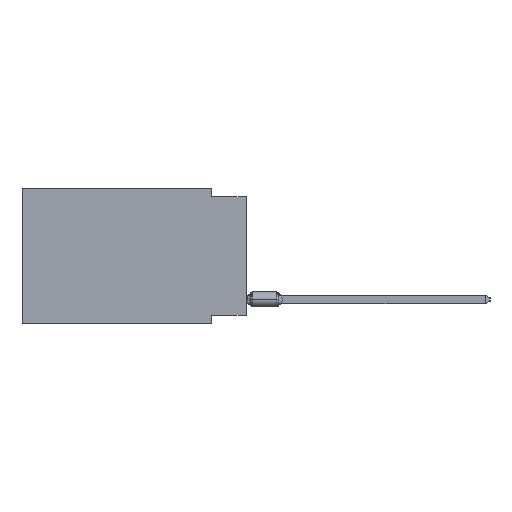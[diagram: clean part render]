
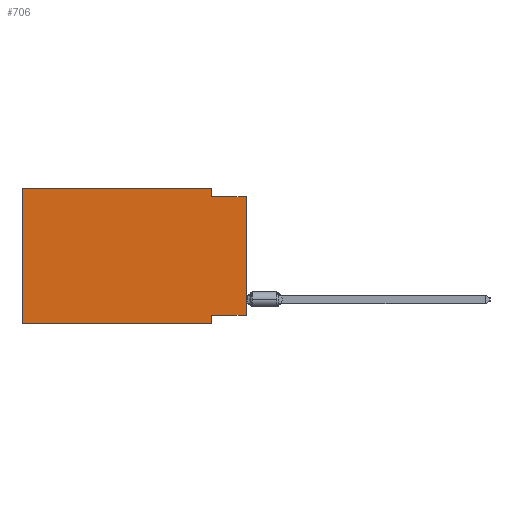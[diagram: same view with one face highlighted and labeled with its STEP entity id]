
A CAD part, left-side view. The second image highlights one B-rep face of the part: STEP entity #706.
In plain terms, the highlighted planar face has unit normal (-1, 0, 0).
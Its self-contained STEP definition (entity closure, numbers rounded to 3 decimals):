
#706 = ADVANCED_FACE ( 'NONE', ( #7351 ), #43498, .F. ) ;
#986 = EDGE_CURVE ( 'NONE', #22717, #11102, #21103, .T. ) ;
#1200 = DIRECTION ( 'NONE',  ( 0., -1., 0. ) ) ;
#1760 = CARTESIAN_POINT ( 'NONE',  ( 0., 2.54, -9.906 ) ) ;
#1798 = VECTOR ( 'NONE', #3731, 1000. ) ;
#3317 = EDGE_CURVE ( 'NONE', #22717, #34356, #41170, .T. ) ;
#3731 = DIRECTION ( 'NONE',  ( 0., 0., -1. ) ) ;
#3809 = ORIENTED_EDGE ( 'NONE', *, *, #32421, .T. ) ;
#5540 = VERTEX_POINT ( 'NONE', #10355 ) ;
#5563 = VECTOR ( 'NONE', #15455, 1000. ) ;
#6187 = EDGE_CURVE ( 'NONE', #42381, #5540, #33834, .T. ) ;
#7033 = LINE ( 'NONE', #28696, #10591 ) ;
#7082 = CARTESIAN_POINT ( 'NONE',  ( 0., 0., -9.271 ) ) ;
#7111 = EDGE_CURVE ( 'NONE', #15736, #25233, #12477, .T. ) ;
#7320 = CARTESIAN_POINT ( 'NONE',  ( 0., 2.54, 0. ) ) ;
#7351 = FACE_OUTER_BOUND ( 'NONE', #18361, .T. ) ;
#9083 = ORIENTED_EDGE ( 'NONE', *, *, #23243, .F. ) ;
#9241 = AXIS2_PLACEMENT_3D ( 'NONE', #39931, #40633, #32341 ) ;
#9351 = ORIENTED_EDGE ( 'NONE', *, *, #14337, .F. ) ;
#9689 = ORIENTED_EDGE ( 'NONE', *, *, #29001, .F. ) ;
#10355 = CARTESIAN_POINT ( 'NONE',  ( 0., 0., -0.635 ) ) ;
#10515 = ORIENTED_EDGE ( 'NONE', *, *, #6187, .F. ) ;
#10591 = VECTOR ( 'NONE', #32966, 1000. ) ;
#11102 = VERTEX_POINT ( 'NONE', #21456 ) ;
#11658 = LINE ( 'NONE', #18789, #5563 ) ;
#11921 = CARTESIAN_POINT ( 'NONE',  ( 0., 16.383, -9.906 ) ) ;
#12477 = LINE ( 'NONE', #7082, #19627 ) ;
#12987 = ORIENTED_EDGE ( 'NONE', *, *, #7111, .F. ) ;
#13678 = VECTOR ( 'NONE', #1200, 1000. ) ;
#14337 = EDGE_CURVE ( 'NONE', #11102, #37100, #11658, .T. ) ;
#15455 = DIRECTION ( 'NONE',  ( 0., -1., 0. ) ) ;
#15736 = VERTEX_POINT ( 'NONE', #16177 ) ;
#16177 = CARTESIAN_POINT ( 'NONE',  ( 0., 0., -9.271 ) ) ;
#16295 = DIRECTION ( 'NONE',  ( 0., 0., -1. ) ) ;
#16545 = VECTOR ( 'NONE', #37151, 1000. ) ;
#18216 = ORIENTED_EDGE ( 'NONE', *, *, #986, .F. ) ;
#18361 = EDGE_LOOP ( 'NONE', ( #3809, #10515, #9689, #9351, #18216, #40103, #9083, #12987 ) ) ;
#18789 = CARTESIAN_POINT ( 'NONE',  ( 0., 16.383, 0. ) ) ;
#19627 = VECTOR ( 'NONE', #33659, 1000. ) ;
#20380 = CARTESIAN_POINT ( 'NONE',  ( 0., 16.383, 0. ) ) ;
#21103 = LINE ( 'NONE', #20380, #34344 ) ;
#21456 = CARTESIAN_POINT ( 'NONE',  ( 0., 16.383, 0. ) ) ;
#21827 = LINE ( 'NONE', #36335, #1798 ) ;
#22060 = CARTESIAN_POINT ( 'NONE',  ( 0., 16.383, -9.906 ) ) ;
#22717 = VERTEX_POINT ( 'NONE', #22060 ) ;
#23243 = EDGE_CURVE ( 'NONE', #25233, #34356, #45064, .T. ) ;
#25233 = VERTEX_POINT ( 'NONE', #34062 ) ;
#27772 = DIRECTION ( 'NONE',  ( 0., 0., 1. ) ) ;
#28696 = CARTESIAN_POINT ( 'NONE',  ( 0., 0., 0. ) ) ;
#29001 = EDGE_CURVE ( 'NONE', #37100, #42381, #21827, .T. ) ;
#32341 = DIRECTION ( 'NONE',  ( 0., 0., -1. ) ) ;
#32421 = EDGE_CURVE ( 'NONE', #15736, #5540, #7033, .T. ) ;
#32966 = DIRECTION ( 'NONE',  ( 0., 0., 1. ) ) ;
#33659 = DIRECTION ( 'NONE',  ( 0., 1., 0. ) ) ;
#33834 = LINE ( 'NONE', #40947, #16545 ) ;
#34062 = CARTESIAN_POINT ( 'NONE',  ( 0., 2.54, -9.271 ) ) ;
#34189 = VECTOR ( 'NONE', #16295, 1000. ) ;
#34344 = VECTOR ( 'NONE', #27772, 1000. ) ;
#34356 = VERTEX_POINT ( 'NONE', #46324 ) ;
#36335 = CARTESIAN_POINT ( 'NONE',  ( 0., 2.54, 0. ) ) ;
#37100 = VERTEX_POINT ( 'NONE', #7320 ) ;
#37151 = DIRECTION ( 'NONE',  ( 0., -1., 0. ) ) ;
#39931 = CARTESIAN_POINT ( 'NONE',  ( 0., 16.383, 0. ) ) ;
#40103 = ORIENTED_EDGE ( 'NONE', *, *, #3317, .T. ) ;
#40633 = DIRECTION ( 'NONE',  ( 1., 0., 0. ) ) ;
#40947 = CARTESIAN_POINT ( 'NONE',  ( 0., 0., -0.635 ) ) ;
#41170 = LINE ( 'NONE', #11921, #13678 ) ;
#41812 = CARTESIAN_POINT ( 'NONE',  ( 0., 2.54, -0.635 ) ) ;
#42381 = VERTEX_POINT ( 'NONE', #41812 ) ;
#43498 = PLANE ( 'NONE',  #9241 ) ;
#45064 = LINE ( 'NONE', #1760, #34189 ) ;
#46324 = CARTESIAN_POINT ( 'NONE',  ( 0., 2.54, -9.906 ) ) ;
